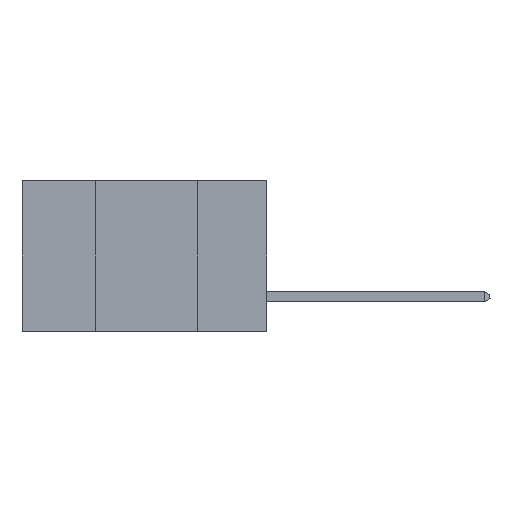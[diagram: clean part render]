
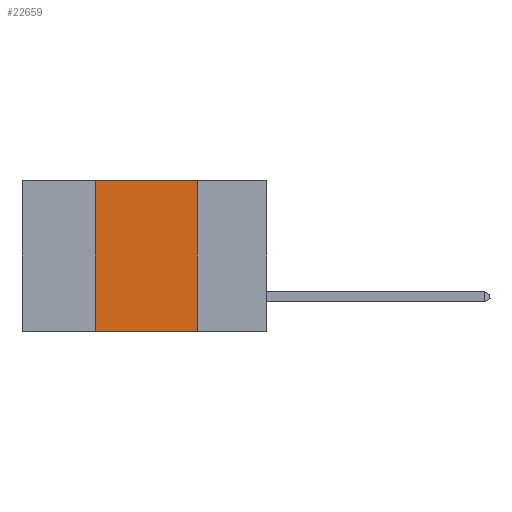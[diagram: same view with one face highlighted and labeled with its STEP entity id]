
A CAD part, left-side view. The second image highlights one B-rep face of the part: STEP entity #22659.
In plain terms, the highlighted planar face has unit normal (-1, 0, 0).
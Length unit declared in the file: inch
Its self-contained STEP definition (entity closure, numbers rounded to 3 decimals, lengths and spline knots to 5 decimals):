
#1766 = PLANE ( 'NONE',  #16459 ) ;
#1901 = ORIENTED_EDGE ( 'NONE', *, *, #9187, .F. ) ;
#2760 = CARTESIAN_POINT ( 'NONE',  ( 0., 0.17, -0.37 ) ) ;
#3188 = LINE ( 'NONE', #23486, #14442 ) ;
#3395 = EDGE_CURVE ( 'NONE', #13563, #13889, #10412, .T. ) ;
#4880 = VECTOR ( 'NONE', #18538, 39.37008 ) ;
#5816 = ORIENTED_EDGE ( 'NONE', *, *, #27728, .F. ) ;
#6070 = CARTESIAN_POINT ( 'NONE',  ( 0., 0.42, 0. ) ) ;
#8333 = VERTEX_POINT ( 'NONE', #26471 ) ;
#9187 = EDGE_CURVE ( 'NONE', #13563, #13049, #25871, .T. ) ;
#9848 = LINE ( 'NONE', #16266, #4880 ) ;
#10386 = FACE_OUTER_BOUND ( 'NONE', #20082, .T. ) ;
#10412 = LINE ( 'NONE', #10786, #22747 ) ;
#10786 = CARTESIAN_POINT ( 'NONE',  ( 0., 0.6, -0.37 ) ) ;
#10827 = CARTESIAN_POINT ( 'NONE',  ( 0., 0.6, 0. ) ) ;
#11582 = EDGE_CURVE ( 'NONE', #8333, #13889, #3188, .T. ) ;
#12983 = DIRECTION ( 'NONE',  ( 1., 0., 0. ) ) ;
#13049 = VERTEX_POINT ( 'NONE', #13163 ) ;
#13163 = CARTESIAN_POINT ( 'NONE',  ( 0., 0.42, 0. ) ) ;
#13563 = VERTEX_POINT ( 'NONE', #28100 ) ;
#13751 = ORIENTED_EDGE ( 'NONE', *, *, #11582, .F. ) ;
#13827 = VECTOR ( 'NONE', #26490, 39.37008 ) ;
#13889 = VERTEX_POINT ( 'NONE', #2760 ) ;
#14442 = VECTOR ( 'NONE', #18726, 39.37008 ) ;
#16266 = CARTESIAN_POINT ( 'NONE',  ( 0., 0.6, 0. ) ) ;
#16459 = AXIS2_PLACEMENT_3D ( 'NONE', #10827, #12983, #17324 ) ;
#17324 = DIRECTION ( 'NONE',  ( 0., 0., -1. ) ) ;
#18538 = DIRECTION ( 'NONE',  ( 0., -1., 0. ) ) ;
#18726 = DIRECTION ( 'NONE',  ( 0., 0., -1. ) ) ;
#20082 = EDGE_LOOP ( 'NONE', ( #13751, #5816, #1901, #22899 ) ) ;
#21871 = DIRECTION ( 'NONE',  ( 0., -1., 0. ) ) ;
#22659 = ADVANCED_FACE ( 'NONE', ( #10386 ), #1766, .F. ) ;
#22747 = VECTOR ( 'NONE', #21871, 39.37008 ) ;
#22899 = ORIENTED_EDGE ( 'NONE', *, *, #3395, .T. ) ;
#23486 = CARTESIAN_POINT ( 'NONE',  ( 0., 0.17, 0. ) ) ;
#25871 = LINE ( 'NONE', #6070, #13827 ) ;
#26471 = CARTESIAN_POINT ( 'NONE',  ( 0., 0.17, 0. ) ) ;
#26490 = DIRECTION ( 'NONE',  ( 0., 0., 1. ) ) ;
#27728 = EDGE_CURVE ( 'NONE', #13049, #8333, #9848, .T. ) ;
#28100 = CARTESIAN_POINT ( 'NONE',  ( 0., 0.42, -0.37 ) ) ;
